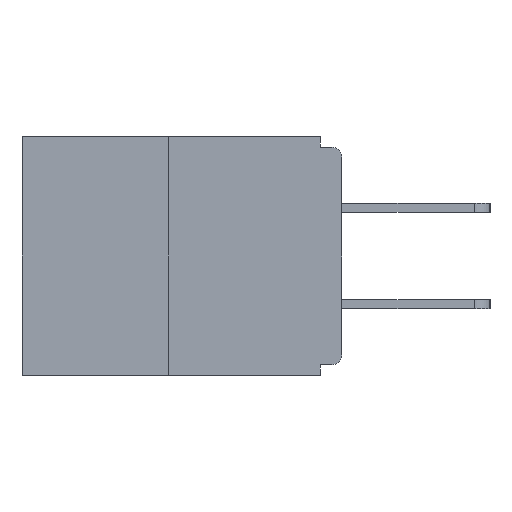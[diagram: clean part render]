
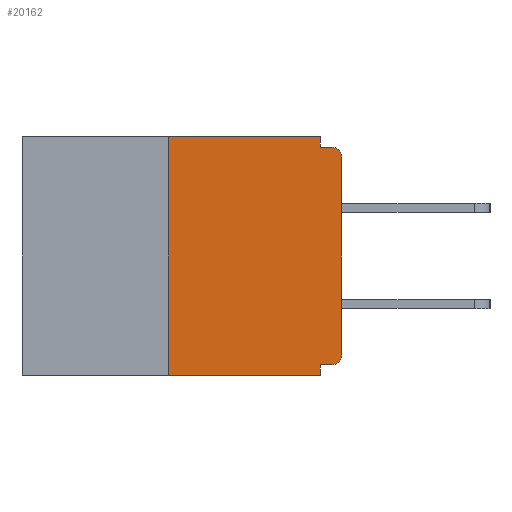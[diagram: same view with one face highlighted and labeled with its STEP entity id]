
A CAD part, left-side view. The second image highlights one B-rep face of the part: STEP entity #20162.
In plain terms, the highlighted planar face has unit normal (-1, 0, 0).
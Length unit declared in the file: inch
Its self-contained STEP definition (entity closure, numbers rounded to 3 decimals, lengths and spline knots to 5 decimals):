
#941 = CARTESIAN_POINT ( 'NONE',  ( 0., 0.031, 0. ) ) ;
#1009 = EDGE_CURVE ( 'NONE', #21023, #3248, #6090, .T. ) ;
#1012 = CARTESIAN_POINT ( 'NONE',  ( 0., 0.031, -0.343 ) ) ;
#1142 = CIRCLE ( 'NONE', #27530, 0.015 ) ;
#1437 = CARTESIAN_POINT ( 'NONE',  ( 0., 0.015, -0.03 ) ) ;
#1709 = EDGE_CURVE ( 'NONE', #13999, #21495, #2931, .T. ) ;
#2251 = CARTESIAN_POINT ( 'NONE',  ( 0., 0.031, -0.015 ) ) ;
#2931 = LINE ( 'NONE', #5965, #16982 ) ;
#2978 = VECTOR ( 'NONE', #26988, 39.37008 ) ;
#3018 = DIRECTION ( 'NONE',  ( 0., 0., -1. ) ) ;
#3105 = DIRECTION ( 'NONE',  ( 0., 1., 0. ) ) ;
#3248 = VERTEX_POINT ( 'NONE', #13023 ) ;
#3361 = DIRECTION ( 'NONE',  ( 1., 0., 0. ) ) ;
#3405 = VERTEX_POINT ( 'NONE', #13505 ) ;
#3629 = DIRECTION ( 'NONE',  ( -1., 0., 0. ) ) ;
#3711 = LINE ( 'NONE', #24902, #14003 ) ;
#4412 = ORIENTED_EDGE ( 'NONE', *, *, #9215, .T. ) ;
#4472 = VECTOR ( 'NONE', #3018, 39.37008 ) ;
#4892 = CIRCLE ( 'NONE', #14928, 0.015 ) ;
#5477 = CARTESIAN_POINT ( 'NONE',  ( 0., 0.015, -0.313 ) ) ;
#5750 = DIRECTION ( 'NONE',  ( 0., 0., -1. ) ) ;
#5783 = CARTESIAN_POINT ( 'NONE',  ( 0., 0., 0. ) ) ;
#5965 = CARTESIAN_POINT ( 'NONE',  ( 0., 0.46, -0.343 ) ) ;
#6047 = VECTOR ( 'NONE', #10185, 39.37008 ) ;
#6090 = LINE ( 'NONE', #26775, #20803 ) ;
#6521 = EDGE_CURVE ( 'NONE', #26155, #21894, #3711, .T. ) ;
#7025 = VECTOR ( 'NONE', #27874, 39.37008 ) ;
#7057 = ORIENTED_EDGE ( 'NONE', *, *, #6521, .F. ) ;
#8100 = ORIENTED_EDGE ( 'NONE', *, *, #14045, .F. ) ;
#8878 = EDGE_CURVE ( 'NONE', #23539, #18992, #26690, .T. ) ;
#9215 = EDGE_CURVE ( 'NONE', #11723, #3405, #18384, .T. ) ;
#9291 = ORIENTED_EDGE ( 'NONE', *, *, #8878, .F. ) ;
#9846 = ORIENTED_EDGE ( 'NONE', *, *, #1709, .T. ) ;
#10185 = DIRECTION ( 'NONE',  ( 0., 0., 1. ) ) ;
#11456 = LINE ( 'NONE', #21083, #7025 ) ;
#11723 = VERTEX_POINT ( 'NONE', #14025 ) ;
#11804 = CARTESIAN_POINT ( 'NONE',  ( 0., 0.46, 0. ) ) ;
#12097 = DIRECTION ( 'NONE',  ( 0., 0., -1. ) ) ;
#12246 = CARTESIAN_POINT ( 'NONE',  ( 0., 0.25, 0. ) ) ;
#12593 = ORIENTED_EDGE ( 'NONE', *, *, #21255, .T. ) ;
#12882 = DIRECTION ( 'NONE',  ( 0., 0., -1. ) ) ;
#12922 = CARTESIAN_POINT ( 'NONE',  ( 0., 0.015, -0.328 ) ) ;
#13023 = CARTESIAN_POINT ( 'NONE',  ( 0., 0.015, -0.015 ) ) ;
#13286 = CARTESIAN_POINT ( 'NONE',  ( 0., 0.031, -0.343 ) ) ;
#13505 = CARTESIAN_POINT ( 'NONE',  ( 0., 0., -0.03 ) ) ;
#13999 = VERTEX_POINT ( 'NONE', #27409 ) ;
#14003 = VECTOR ( 'NONE', #3105, 39.37008 ) ;
#14025 = CARTESIAN_POINT ( 'NONE',  ( 0., 0., -0.313 ) ) ;
#14045 = EDGE_CURVE ( 'NONE', #21894, #21495, #27154, .T. ) ;
#14215 = VECTOR ( 'NONE', #12882, 39.37008 ) ;
#14270 = DIRECTION ( 'NONE',  ( -1., 0., 0. ) ) ;
#14928 = AXIS2_PLACEMENT_3D ( 'NONE', #5477, #14270, #5750 ) ;
#16445 = ORIENTED_EDGE ( 'NONE', *, *, #20824, .F. ) ;
#16982 = VECTOR ( 'NONE', #17350, 39.37008 ) ;
#17350 = DIRECTION ( 'NONE',  ( 0., -1., 0. ) ) ;
#18253 = ORIENTED_EDGE ( 'NONE', *, *, #27075, .F. ) ;
#18384 = LINE ( 'NONE', #5783, #6047 ) ;
#18992 = VERTEX_POINT ( 'NONE', #941 ) ;
#19435 = DIRECTION ( 'NONE',  ( 0., 0., -1. ) ) ;
#20162 = ADVANCED_FACE ( 'NONE', ( #24235 ), #27564, .F. ) ;
#20302 = AXIS2_PLACEMENT_3D ( 'NONE', #27466, #3361, #12097 ) ;
#20803 = VECTOR ( 'NONE', #24934, 39.37008 ) ;
#20824 = EDGE_CURVE ( 'NONE', #18992, #21023, #23491, .T. ) ;
#20940 = ORIENTED_EDGE ( 'NONE', *, *, #1009, .F. ) ;
#21023 = VERTEX_POINT ( 'NONE', #2251 ) ;
#21083 = CARTESIAN_POINT ( 'NONE',  ( 0., 0.25, 0. ) ) ;
#21255 = EDGE_CURVE ( 'NONE', #3405, #3248, #1142, .T. ) ;
#21269 = ORIENTED_EDGE ( 'NONE', *, *, #27679, .T. ) ;
#21495 = VERTEX_POINT ( 'NONE', #13286 ) ;
#21804 = CARTESIAN_POINT ( 'NONE',  ( 0., 0.031, -0.328 ) ) ;
#21894 = VERTEX_POINT ( 'NONE', #21804 ) ;
#22058 = EDGE_LOOP ( 'NONE', ( #9291, #18253, #9846, #8100, #7057, #21269, #4412, #12593, #20940, #16445 ) ) ;
#23491 = LINE ( 'NONE', #25993, #14215 ) ;
#23539 = VERTEX_POINT ( 'NONE', #12246 ) ;
#24235 = FACE_OUTER_BOUND ( 'NONE', #22058, .T. ) ;
#24902 = CARTESIAN_POINT ( 'NONE',  ( 0., 0., -0.328 ) ) ;
#24934 = DIRECTION ( 'NONE',  ( 0., -1., 0. ) ) ;
#25993 = CARTESIAN_POINT ( 'NONE',  ( 0., 0.031, 0. ) ) ;
#26155 = VERTEX_POINT ( 'NONE', #12922 ) ;
#26690 = LINE ( 'NONE', #11804, #2978 ) ;
#26775 = CARTESIAN_POINT ( 'NONE',  ( 0., 0., -0.015 ) ) ;
#26988 = DIRECTION ( 'NONE',  ( 0., -1., 0. ) ) ;
#27075 = EDGE_CURVE ( 'NONE', #13999, #23539, #11456, .T. ) ;
#27154 = LINE ( 'NONE', #1012, #4472 ) ;
#27409 = CARTESIAN_POINT ( 'NONE',  ( 0., 0.25, -0.343 ) ) ;
#27466 = CARTESIAN_POINT ( 'NONE',  ( 0., 0.46, 0. ) ) ;
#27530 = AXIS2_PLACEMENT_3D ( 'NONE', #1437, #3629, #19435 ) ;
#27564 = PLANE ( 'NONE',  #20302 ) ;
#27679 = EDGE_CURVE ( 'NONE', #26155, #11723, #4892, .T. ) ;
#27874 = DIRECTION ( 'NONE',  ( 0., 0., 1. ) ) ;
